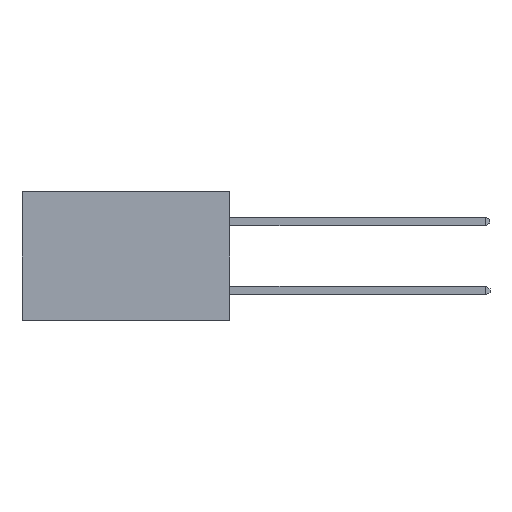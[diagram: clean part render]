
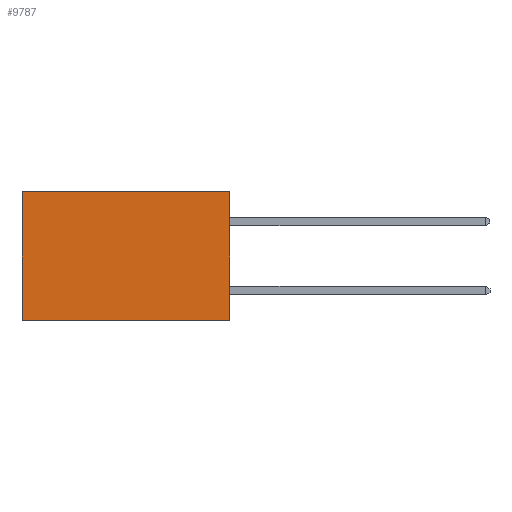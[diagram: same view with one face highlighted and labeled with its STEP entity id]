
A CAD part, left-side view. The second image highlights one B-rep face of the part: STEP entity #9787.
In plain terms, the highlighted planar face has unit normal (-1, 0, 0).
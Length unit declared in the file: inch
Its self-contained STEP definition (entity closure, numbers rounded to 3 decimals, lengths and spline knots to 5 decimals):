
#6 = DIRECTION ( 'NONE',  ( 0., 0., -1. ) ) ;
#269 = VECTOR ( 'NONE', #4823, 39.37008 ) ;
#621 = EDGE_CURVE ( 'NONE', #1209, #3579, #5252, .T. ) ;
#699 = VERTEX_POINT ( 'NONE', #844 ) ;
#734 = LINE ( 'NONE', #7726, #5163 ) ;
#826 = EDGE_CURVE ( 'NONE', #3579, #699, #5655, .T. ) ;
#844 = CARTESIAN_POINT ( 'NONE',  ( 0.2615, 0.6, -0.37 ) ) ;
#1209 = VERTEX_POINT ( 'NONE', #10716 ) ;
#1467 = AXIS2_PLACEMENT_3D ( 'NONE', #8733, #5323, #6 ) ;
#1526 = FACE_OUTER_BOUND ( 'NONE', #9126, .T. ) ;
#2269 = EDGE_CURVE ( 'NONE', #3742, #699, #11045, .T. ) ;
#2344 = ORIENTED_EDGE ( 'NONE', *, *, #621, .T. ) ;
#3579 = VERTEX_POINT ( 'NONE', #7771 ) ;
#3712 = CARTESIAN_POINT ( 'NONE',  ( 0.2615, 0., -0.37 ) ) ;
#3742 = VERTEX_POINT ( 'NONE', #3712 ) ;
#3811 = ORIENTED_EDGE ( 'NONE', *, *, #826, .T. ) ;
#4121 = DIRECTION ( 'NONE',  ( 0., 1., 0. ) ) ;
#4383 = CARTESIAN_POINT ( 'NONE',  ( 0.2615, 0., -0.37 ) ) ;
#4435 = ORIENTED_EDGE ( 'NONE', *, *, #2269, .F. ) ;
#4653 = DIRECTION ( 'NONE',  ( 0., 0., -1. ) ) ;
#4823 = DIRECTION ( 'NONE',  ( 0., 1., 0. ) ) ;
#5163 = VECTOR ( 'NONE', #7872, 39.37008 ) ;
#5252 = LINE ( 'NONE', #6117, #269 ) ;
#5323 = DIRECTION ( 'NONE',  ( 1., 0., 0. ) ) ;
#5574 = CARTESIAN_POINT ( 'NONE',  ( 0.2615, 0.6, -0.37 ) ) ;
#5655 = LINE ( 'NONE', #5574, #7402 ) ;
#6117 = CARTESIAN_POINT ( 'NONE',  ( 0.2615, 0., 0. ) ) ;
#6121 = EDGE_CURVE ( 'NONE', #1209, #3742, #734, .T. ) ;
#7402 = VECTOR ( 'NONE', #4653, 39.37008 ) ;
#7726 = CARTESIAN_POINT ( 'NONE',  ( 0.2615, 0., -0.37 ) ) ;
#7771 = CARTESIAN_POINT ( 'NONE',  ( 0.2615, 0.6, 0. ) ) ;
#7872 = DIRECTION ( 'NONE',  ( 0., 0., -1. ) ) ;
#8208 = ORIENTED_EDGE ( 'NONE', *, *, #6121, .F. ) ;
#8733 = CARTESIAN_POINT ( 'NONE',  ( 0.2615, 0., -0.37 ) ) ;
#9126 = EDGE_LOOP ( 'NONE', ( #3811, #4435, #8208, #2344 ) ) ;
#9520 = PLANE ( 'NONE',  #1467 ) ;
#9787 = ADVANCED_FACE ( 'NONE', ( #1526 ), #9520, .F. ) ;
#10716 = CARTESIAN_POINT ( 'NONE',  ( 0.2615, 0., 0. ) ) ;
#10810 = VECTOR ( 'NONE', #4121, 39.37008 ) ;
#11045 = LINE ( 'NONE', #4383, #10810 ) ;
